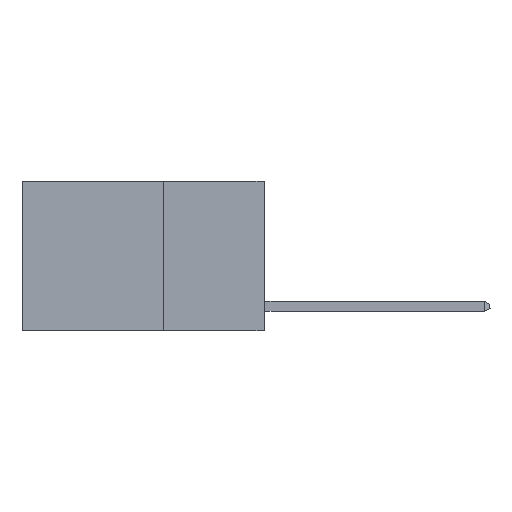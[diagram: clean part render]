
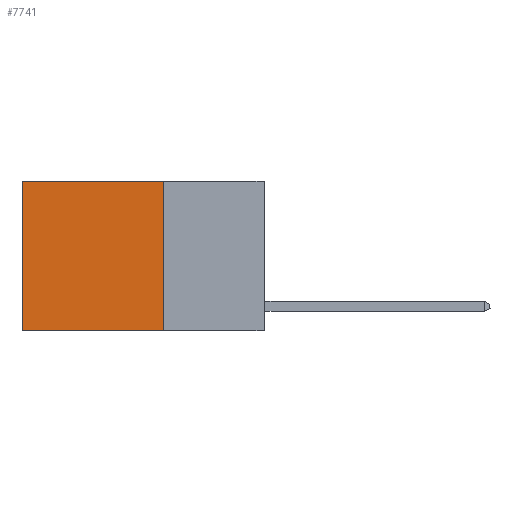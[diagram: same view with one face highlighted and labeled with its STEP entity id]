
A CAD part, left-side view. The second image highlights one B-rep face of the part: STEP entity #7741.
In plain terms, the highlighted planar face has unit normal (-1, 0, 0).
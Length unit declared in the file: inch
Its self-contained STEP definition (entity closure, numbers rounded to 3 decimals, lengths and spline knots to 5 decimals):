
#498 = LINE ( 'NONE', #9814, #2844 ) ;
#576 = CARTESIAN_POINT ( 'NONE',  ( 0.2625, 0.6, 0. ) ) ;
#609 = VERTEX_POINT ( 'NONE', #2114 ) ;
#719 = DIRECTION ( 'NONE',  ( 1., 0., 0. ) ) ;
#780 = CARTESIAN_POINT ( 'NONE',  ( 0.2625, 0.6, 0. ) ) ;
#793 = VERTEX_POINT ( 'NONE', #780 ) ;
#1217 = ORIENTED_EDGE ( 'NONE', *, *, #5168, .T. ) ;
#1642 = DIRECTION ( 'NONE',  ( 0., 0., -1. ) ) ;
#2114 = CARTESIAN_POINT ( 'NONE',  ( 0.2625, 0.25, 0. ) ) ;
#2256 = EDGE_CURVE ( 'NONE', #6292, #11832, #5523, .T. ) ;
#2373 = LINE ( 'NONE', #10684, #5444 ) ;
#2427 = DIRECTION ( 'NONE',  ( 0., 1., 0. ) ) ;
#2436 = DIRECTION ( 'NONE',  ( 0., 0., -1. ) ) ;
#2464 = CARTESIAN_POINT ( 'NONE',  ( 0.2625, 0.25, -0.37 ) ) ;
#2844 = VECTOR ( 'NONE', #1642, 39.37008 ) ;
#3387 = VECTOR ( 'NONE', #5587, 39.37008 ) ;
#3441 = PLANE ( 'NONE',  #10541 ) ;
#3975 = CARTESIAN_POINT ( 'NONE',  ( 0.2625, 0.6, -0.37 ) ) ;
#4362 = FACE_OUTER_BOUND ( 'NONE', #10391, .T. ) ;
#5168 = EDGE_CURVE ( 'NONE', #609, #793, #2373, .T. ) ;
#5316 = CARTESIAN_POINT ( 'NONE',  ( 0.2625, 0.25, 0. ) ) ;
#5444 = VECTOR ( 'NONE', #2427, 39.37008 ) ;
#5523 = LINE ( 'NONE', #7252, #3387 ) ;
#5587 = DIRECTION ( 'NONE',  ( 0., 1., 0. ) ) ;
#5840 = DIRECTION ( 'NONE',  ( 0., 0., -1. ) ) ;
#5987 = EDGE_CURVE ( 'NONE', #609, #6292, #498, .T. ) ;
#6292 = VERTEX_POINT ( 'NONE', #2464 ) ;
#6644 = ORIENTED_EDGE ( 'NONE', *, *, #5987, .F. ) ;
#7218 = EDGE_CURVE ( 'NONE', #793, #11832, #8710, .T. ) ;
#7252 = CARTESIAN_POINT ( 'NONE',  ( 0.2625, 0.25, -0.37 ) ) ;
#7741 = ADVANCED_FACE ( 'NONE', ( #4362 ), #3441, .F. ) ;
#8710 = LINE ( 'NONE', #576, #11659 ) ;
#9814 = CARTESIAN_POINT ( 'NONE',  ( 0.2625, 0.25, 0. ) ) ;
#10380 = ORIENTED_EDGE ( 'NONE', *, *, #7218, .T. ) ;
#10391 = EDGE_LOOP ( 'NONE', ( #10380, #11773, #6644, #1217 ) ) ;
#10541 = AXIS2_PLACEMENT_3D ( 'NONE', #5316, #719, #5840 ) ;
#10684 = CARTESIAN_POINT ( 'NONE',  ( 0.2625, 0.25, 0. ) ) ;
#11659 = VECTOR ( 'NONE', #2436, 39.37008 ) ;
#11773 = ORIENTED_EDGE ( 'NONE', *, *, #2256, .F. ) ;
#11832 = VERTEX_POINT ( 'NONE', #3975 ) ;
